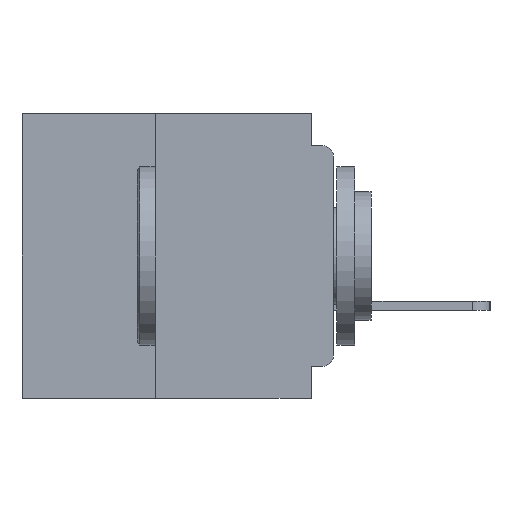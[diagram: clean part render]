
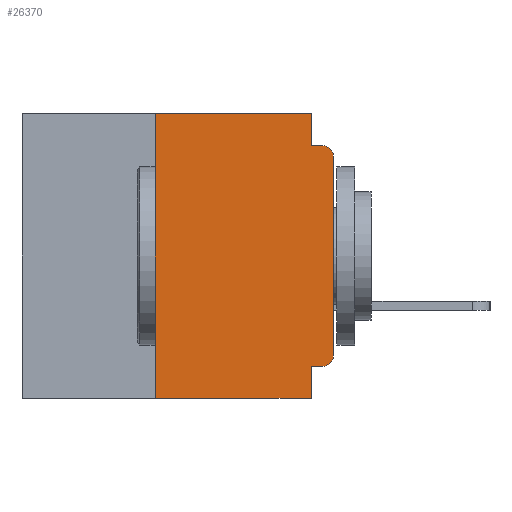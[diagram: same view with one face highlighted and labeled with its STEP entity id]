
A CAD part, left-side view. The second image highlights one B-rep face of the part: STEP entity #26370.
In plain terms, the highlighted planar face has unit normal (-1, 0, 0).
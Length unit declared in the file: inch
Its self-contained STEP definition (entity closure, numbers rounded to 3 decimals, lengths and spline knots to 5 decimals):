
#73 = EDGE_CURVE ( 'NONE', #6671, #9248, #20713, .T. ) ;
#303 = ORIENTED_EDGE ( 'NONE', *, *, #18312, .F. ) ;
#2271 = EDGE_CURVE ( 'NONE', #3463, #6671, #6666, .T. ) ;
#2834 = CARTESIAN_POINT ( 'NONE',  ( 0., 0.015, -0.045 ) ) ;
#3463 = VERTEX_POINT ( 'NONE', #20757 ) ;
#5061 = CARTESIAN_POINT ( 'NONE',  ( 0., 0.031, -0.355 ) ) ;
#5539 = DIRECTION ( 'NONE',  ( 0., 0., -1. ) ) ;
#5661 = DIRECTION ( 'NONE',  ( 0., 0., -1. ) ) ;
#6059 = CARTESIAN_POINT ( 'NONE',  ( 0., 0.015, -0.34 ) ) ;
#6666 = LINE ( 'NONE', #11998, #20541 ) ;
#6671 = VERTEX_POINT ( 'NONE', #20182 ) ;
#7014 = CARTESIAN_POINT ( 'NONE',  ( 0., 0.031, 0. ) ) ;
#7116 = EDGE_CURVE ( 'NONE', #8468, #29343, #31088, .T. ) ;
#7622 = FACE_OUTER_BOUND ( 'NONE', #23718, .T. ) ;
#8432 = VERTEX_POINT ( 'NONE', #25806 ) ;
#8468 = VERTEX_POINT ( 'NONE', #31583 ) ;
#8498 = VERTEX_POINT ( 'NONE', #12275 ) ;
#8876 = DIRECTION ( 'NONE',  ( 0., 0., -1. ) ) ;
#9248 = VERTEX_POINT ( 'NONE', #7014 ) ;
#9579 = VECTOR ( 'NONE', #24201, 39.37008 ) ;
#9829 = ORIENTED_EDGE ( 'NONE', *, *, #18628, .T. ) ;
#9914 = LINE ( 'NONE', #16791, #23835 ) ;
#10101 = EDGE_CURVE ( 'NONE', #8498, #8468, #24377, .T. ) ;
#10177 = ORIENTED_EDGE ( 'NONE', *, *, #73, .F. ) ;
#10379 = CARTESIAN_POINT ( 'NONE',  ( 0., 0., -0.355 ) ) ;
#11702 = LINE ( 'NONE', #10379, #25651 ) ;
#11734 = LINE ( 'NONE', #22327, #17393 ) ;
#11873 = DIRECTION ( 'NONE',  ( 0., 0., 1. ) ) ;
#11998 = CARTESIAN_POINT ( 'NONE',  ( 0., 0.25, -0.4 ) ) ;
#12072 = ORIENTED_EDGE ( 'NONE', *, *, #34902, .F. ) ;
#12082 = ORIENTED_EDGE ( 'NONE', *, *, #7116, .T. ) ;
#12275 = CARTESIAN_POINT ( 'NONE',  ( 0., 0., -0.34 ) ) ;
#12521 = AXIS2_PLACEMENT_3D ( 'NONE', #6059, #25527, #8876 ) ;
#13448 = VECTOR ( 'NONE', #15364, 39.37008 ) ;
#14343 = LINE ( 'NONE', #34731, #13448 ) ;
#14885 = EDGE_CURVE ( 'NONE', #8432, #8498, #35655, .T. ) ;
#15364 = DIRECTION ( 'NONE',  ( 0., -1., 0. ) ) ;
#16619 = PLANE ( 'NONE',  #29545 ) ;
#16621 = DIRECTION ( 'NONE',  ( -1., 0., 0. ) ) ;
#16791 = CARTESIAN_POINT ( 'NONE',  ( 0., 0., -0.045 ) ) ;
#17033 = DIRECTION ( 'NONE',  ( 0., -1., 0. ) ) ;
#17122 = VERTEX_POINT ( 'NONE', #28118 ) ;
#17164 = VECTOR ( 'NONE', #21026, 39.37008 ) ;
#17247 = DIRECTION ( 'NONE',  ( 0., -1., 0. ) ) ;
#17393 = VECTOR ( 'NONE', #5661, 39.37008 ) ;
#17631 = EDGE_CURVE ( 'NONE', #17122, #29343, #9914, .T. ) ;
#18312 = EDGE_CURVE ( 'NONE', #9248, #17122, #11734, .T. ) ;
#18628 = EDGE_CURVE ( 'NONE', #3463, #30417, #14343, .T. ) ;
#19135 = ORIENTED_EDGE ( 'NONE', *, *, #10101, .T. ) ;
#19207 = ORIENTED_EDGE ( 'NONE', *, *, #14885, .T. ) ;
#19859 = VECTOR ( 'NONE', #17247, 39.37008 ) ;
#20182 = CARTESIAN_POINT ( 'NONE',  ( 0., 0.25, 0. ) ) ;
#20541 = VECTOR ( 'NONE', #11873, 39.37008 ) ;
#20713 = LINE ( 'NONE', #24982, #19859 ) ;
#20757 = CARTESIAN_POINT ( 'NONE',  ( 0., 0.25, -0.4 ) ) ;
#21026 = DIRECTION ( 'NONE',  ( 0., 0., -1. ) ) ;
#21150 = ORIENTED_EDGE ( 'NONE', *, *, #2271, .F. ) ;
#22076 = CARTESIAN_POINT ( 'NONE',  ( 0., 0.437, 0. ) ) ;
#22196 = DIRECTION ( 'NONE',  ( 1., 0., 0. ) ) ;
#22327 = CARTESIAN_POINT ( 'NONE',  ( 0., 0.031, 0. ) ) ;
#23718 = EDGE_LOOP ( 'NONE', ( #19135, #12082, #29171, #303, #10177, #21150, #9829, #12072, #26578, #19207 ) ) ;
#23835 = VECTOR ( 'NONE', #17033, 39.37008 ) ;
#24201 = DIRECTION ( 'NONE',  ( 0., 0., 1. ) ) ;
#24377 = LINE ( 'NONE', #26980, #9579 ) ;
#24982 = CARTESIAN_POINT ( 'NONE',  ( 0., 0.437, 0. ) ) ;
#25527 = DIRECTION ( 'NONE',  ( -1., 0., 0. ) ) ;
#25651 = VECTOR ( 'NONE', #27023, 39.37008 ) ;
#25806 = CARTESIAN_POINT ( 'NONE',  ( 0., 0.015, -0.355 ) ) ;
#26370 = ADVANCED_FACE ( 'NONE', ( #7622 ), #16619, .F. ) ;
#26578 = ORIENTED_EDGE ( 'NONE', *, *, #31679, .F. ) ;
#26980 = CARTESIAN_POINT ( 'NONE',  ( 0., 0., 0. ) ) ;
#27023 = DIRECTION ( 'NONE',  ( 0., 1., 0. ) ) ;
#28004 = VERTEX_POINT ( 'NONE', #5061 ) ;
#28118 = CARTESIAN_POINT ( 'NONE',  ( 0., 0.031, -0.045 ) ) ;
#29171 = ORIENTED_EDGE ( 'NONE', *, *, #17631, .F. ) ;
#29343 = VERTEX_POINT ( 'NONE', #2834 ) ;
#29545 = AXIS2_PLACEMENT_3D ( 'NONE', #22076, #22196, #5539 ) ;
#29571 = AXIS2_PLACEMENT_3D ( 'NONE', #33206, #16621, #35946 ) ;
#30417 = VERTEX_POINT ( 'NONE', #32520 ) ;
#31088 = CIRCLE ( 'NONE', #29571, 0.015 ) ;
#31583 = CARTESIAN_POINT ( 'NONE',  ( 0., 0., -0.06 ) ) ;
#31679 = EDGE_CURVE ( 'NONE', #8432, #28004, #11702, .T. ) ;
#31901 = LINE ( 'NONE', #34796, #17164 ) ;
#32520 = CARTESIAN_POINT ( 'NONE',  ( 0., 0.031, -0.4 ) ) ;
#33206 = CARTESIAN_POINT ( 'NONE',  ( 0., 0.015, -0.06 ) ) ;
#34731 = CARTESIAN_POINT ( 'NONE',  ( 0., 0.437, -0.4 ) ) ;
#34796 = CARTESIAN_POINT ( 'NONE',  ( 0., 0.031, -0.4 ) ) ;
#34902 = EDGE_CURVE ( 'NONE', #28004, #30417, #31901, .T. ) ;
#35655 = CIRCLE ( 'NONE', #12521, 0.015 ) ;
#35946 = DIRECTION ( 'NONE',  ( 0., 0., -1. ) ) ;
